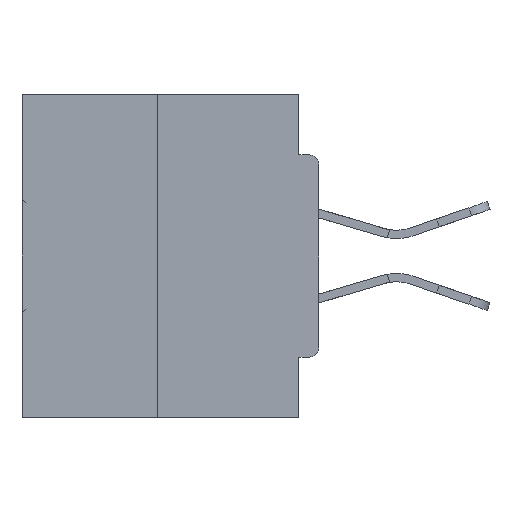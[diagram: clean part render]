
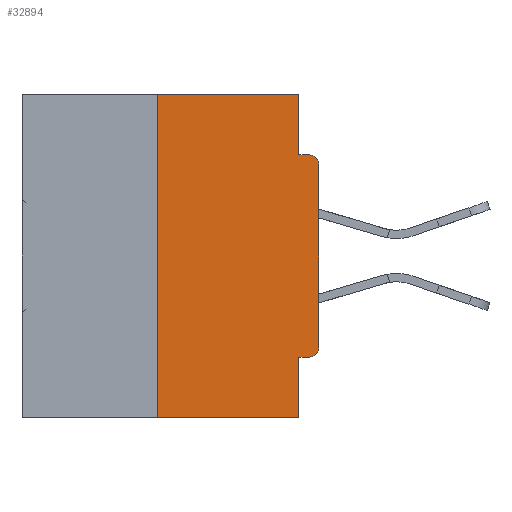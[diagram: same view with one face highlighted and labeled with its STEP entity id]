
A CAD part, left-side view. The second image highlights one B-rep face of the part: STEP entity #32894.
In plain terms, the highlighted planar face has unit normal (-1, 0, 0).
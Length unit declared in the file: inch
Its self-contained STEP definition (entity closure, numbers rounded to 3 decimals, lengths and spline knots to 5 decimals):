
#833 = CARTESIAN_POINT ( 'NONE',  ( 0., 0.031, 0. ) ) ;
#3933 = LINE ( 'NONE', #27232, #14929 ) ;
#4180 = VERTEX_POINT ( 'NONE', #37603 ) ;
#4384 = VECTOR ( 'NONE', #37934, 39.37008 ) ;
#5009 = CARTESIAN_POINT ( 'NONE',  ( 0., 0.25, 0. ) ) ;
#5996 = DIRECTION ( 'NONE',  ( -1., 0., 0. ) ) ;
#6648 = VECTOR ( 'NONE', #21697, 39.37008 ) ;
#6797 = CARTESIAN_POINT ( 'NONE',  ( 0., 0., -0.3915 ) ) ;
#8189 = EDGE_CURVE ( 'NONE', #15523, #12513, #3933, .T. ) ;
#8242 = LINE ( 'NONE', #21109, #6648 ) ;
#8809 = VERTEX_POINT ( 'NONE', #13606 ) ;
#9422 = DIRECTION ( 'NONE',  ( -1., 0., 0. ) ) ;
#9498 = DIRECTION ( 'NONE',  ( 1., 0., 0. ) ) ;
#9825 = EDGE_CURVE ( 'NONE', #8809, #40609, #15811, .T. ) ;
#10059 = ORIENTED_EDGE ( 'NONE', *, *, #18361, .F. ) ;
#10170 = CARTESIAN_POINT ( 'NONE',  ( 0., 0.015, -0.4065 ) ) ;
#10258 = LINE ( 'NONE', #22940, #26896 ) ;
#10877 = AXIS2_PLACEMENT_3D ( 'NONE', #35587, #9498, #42181 ) ;
#11296 = CARTESIAN_POINT ( 'NONE',  ( 0., 0., 0. ) ) ;
#12513 = VERTEX_POINT ( 'NONE', #23250 ) ;
#13276 = LINE ( 'NONE', #5009, #4384 ) ;
#13606 = CARTESIAN_POINT ( 'NONE',  ( 0., 0.031, 0. ) ) ;
#14575 = VERTEX_POINT ( 'NONE', #23465 ) ;
#14929 = VECTOR ( 'NONE', #35551, 39.37008 ) ;
#15501 = AXIS2_PLACEMENT_3D ( 'NONE', #39439, #9422, #42260 ) ;
#15523 = VERTEX_POINT ( 'NONE', #35658 ) ;
#15592 = EDGE_LOOP ( 'NONE', ( #23427, #10059, #32708, #25258, #19162, #15797, #16553, #37595, #19795, #34422 ) ) ;
#15797 = ORIENTED_EDGE ( 'NONE', *, *, #40720, .T. ) ;
#15808 = EDGE_CURVE ( 'NONE', #40609, #41009, #8242, .T. ) ;
#15811 = LINE ( 'NONE', #833, #23077 ) ;
#16072 = DIRECTION ( 'NONE',  ( 0., 0., 1. ) ) ;
#16403 = EDGE_CURVE ( 'NONE', #36593, #15523, #34813, .T. ) ;
#16510 = DIRECTION ( 'NONE',  ( 0., 1., 0. ) ) ;
#16553 = ORIENTED_EDGE ( 'NONE', *, *, #28321, .T. ) ;
#18361 = EDGE_CURVE ( 'NONE', #4180, #32639, #13276, .T. ) ;
#18631 = LINE ( 'NONE', #11296, #21180 ) ;
#18848 = CARTESIAN_POINT ( 'NONE',  ( 0., 0.031, -0.0935 ) ) ;
#19162 = ORIENTED_EDGE ( 'NONE', *, *, #16403, .F. ) ;
#19795 = ORIENTED_EDGE ( 'NONE', *, *, #15808, .F. ) ;
#20739 = CARTESIAN_POINT ( 'NONE',  ( 0., 0.25, 0. ) ) ;
#21109 = CARTESIAN_POINT ( 'NONE',  ( 0., 0., -0.0935 ) ) ;
#21180 = VECTOR ( 'NONE', #16072, 39.37008 ) ;
#21697 = DIRECTION ( 'NONE',  ( 0., -1., 0. ) ) ;
#22564 = VECTOR ( 'NONE', #38727, 39.37008 ) ;
#22940 = CARTESIAN_POINT ( 'NONE',  ( 0., 0.46, -0.5 ) ) ;
#23077 = VECTOR ( 'NONE', #37559, 39.37008 ) ;
#23250 = CARTESIAN_POINT ( 'NONE',  ( 0., 0.031, -0.5 ) ) ;
#23427 = ORIENTED_EDGE ( 'NONE', *, *, #30222, .F. ) ;
#23465 = CARTESIAN_POINT ( 'NONE',  ( 0., 0., -0.1085 ) ) ;
#24950 = CIRCLE ( 'NONE', #15501, 0.015 ) ;
#25258 = ORIENTED_EDGE ( 'NONE', *, *, #8189, .F. ) ;
#26215 = FACE_OUTER_BOUND ( 'NONE', #15592, .T. ) ;
#26896 = VECTOR ( 'NONE', #39432, 39.37008 ) ;
#27099 = EDGE_CURVE ( 'NONE', #14575, #41009, #24950, .T. ) ;
#27232 = CARTESIAN_POINT ( 'NONE',  ( 0., 0.031, -0.5 ) ) ;
#27818 = AXIS2_PLACEMENT_3D ( 'NONE', #42588, #5996, #39345 ) ;
#27822 = VERTEX_POINT ( 'NONE', #6797 ) ;
#28321 = EDGE_CURVE ( 'NONE', #27822, #14575, #18631, .T. ) ;
#28658 = CARTESIAN_POINT ( 'NONE',  ( 0., 0.46, 0. ) ) ;
#29434 = PLANE ( 'NONE',  #10877 ) ;
#30222 = EDGE_CURVE ( 'NONE', #32639, #8809, #31930, .T. ) ;
#31930 = LINE ( 'NONE', #28658, #22564 ) ;
#32639 = VERTEX_POINT ( 'NONE', #20739 ) ;
#32708 = ORIENTED_EDGE ( 'NONE', *, *, #40066, .T. ) ;
#32894 = ADVANCED_FACE ( 'NONE', ( #26215 ), #29434, .F. ) ;
#33203 = VECTOR ( 'NONE', #16510, 39.37008 ) ;
#34422 = ORIENTED_EDGE ( 'NONE', *, *, #9825, .F. ) ;
#34813 = LINE ( 'NONE', #36565, #33203 ) ;
#35551 = DIRECTION ( 'NONE',  ( 0., 0., -1. ) ) ;
#35587 = CARTESIAN_POINT ( 'NONE',  ( 0., 0.46, 0. ) ) ;
#35658 = CARTESIAN_POINT ( 'NONE',  ( 0., 0.031, -0.4065 ) ) ;
#36565 = CARTESIAN_POINT ( 'NONE',  ( 0., 0., -0.4065 ) ) ;
#36593 = VERTEX_POINT ( 'NONE', #10170 ) ;
#37559 = DIRECTION ( 'NONE',  ( 0., 0., -1. ) ) ;
#37595 = ORIENTED_EDGE ( 'NONE', *, *, #27099, .T. ) ;
#37603 = CARTESIAN_POINT ( 'NONE',  ( 0., 0.25, -0.5 ) ) ;
#37934 = DIRECTION ( 'NONE',  ( 0., 0., 1. ) ) ;
#38285 = CARTESIAN_POINT ( 'NONE',  ( 0., 0.015, -0.0935 ) ) ;
#38727 = DIRECTION ( 'NONE',  ( 0., -1., 0. ) ) ;
#39345 = DIRECTION ( 'NONE',  ( 0., 0., -1. ) ) ;
#39432 = DIRECTION ( 'NONE',  ( 0., -1., 0. ) ) ;
#39439 = CARTESIAN_POINT ( 'NONE',  ( 0., 0.015, -0.1085 ) ) ;
#40066 = EDGE_CURVE ( 'NONE', #4180, #12513, #10258, .T. ) ;
#40460 = CIRCLE ( 'NONE', #27818, 0.015 ) ;
#40609 = VERTEX_POINT ( 'NONE', #18848 ) ;
#40720 = EDGE_CURVE ( 'NONE', #36593, #27822, #40460, .T. ) ;
#41009 = VERTEX_POINT ( 'NONE', #38285 ) ;
#42181 = DIRECTION ( 'NONE',  ( 0., 0., -1. ) ) ;
#42260 = DIRECTION ( 'NONE',  ( 0., 0., -1. ) ) ;
#42588 = CARTESIAN_POINT ( 'NONE',  ( 0., 0.015, -0.3915 ) ) ;
